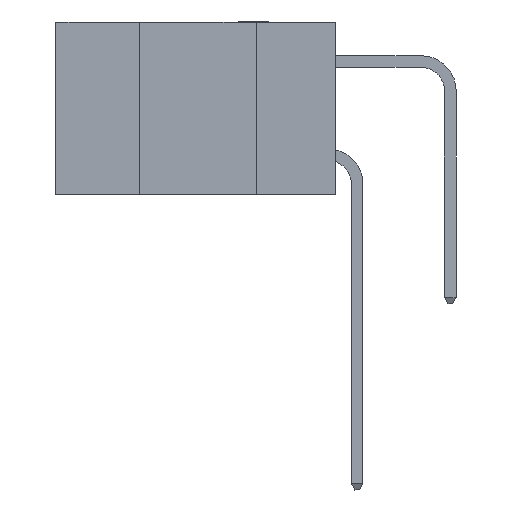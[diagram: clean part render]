
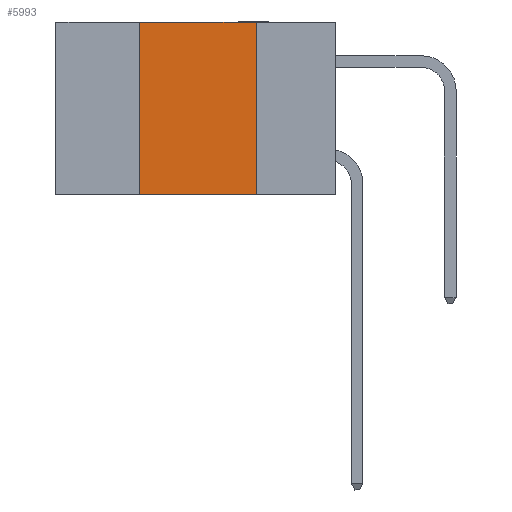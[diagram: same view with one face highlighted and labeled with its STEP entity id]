
A CAD part, left-side view. The second image highlights one B-rep face of the part: STEP entity #5993.
In plain terms, the highlighted planar face has unit normal (-1, 0, 0).
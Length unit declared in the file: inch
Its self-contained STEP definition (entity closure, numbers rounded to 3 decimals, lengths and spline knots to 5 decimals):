
#5 = VECTOR ( 'NONE', #8102, 39.37008 ) ;
#407 = LINE ( 'NONE', #8889, #17826 ) ;
#636 = CARTESIAN_POINT ( 'NONE',  ( 0., 0.6, 0. ) ) ;
#2403 = DIRECTION ( 'NONE',  ( 1., 0., 0. ) ) ;
#3461 = DIRECTION ( 'NONE',  ( 0., 0., 1. ) ) ;
#4046 = CARTESIAN_POINT ( 'NONE',  ( 0., 0.42, 0. ) ) ;
#4615 = VERTEX_POINT ( 'NONE', #21338 ) ;
#4782 = LINE ( 'NONE', #7060, #22530 ) ;
#5993 = ADVANCED_FACE ( 'NONE', ( #9013 ), #21867, .F. ) ;
#6171 = DIRECTION ( 'NONE',  ( 0., -1., 0. ) ) ;
#7060 = CARTESIAN_POINT ( 'NONE',  ( 0., 0.17, 0. ) ) ;
#7502 = VECTOR ( 'NONE', #6171, 39.37008 ) ;
#8099 = VERTEX_POINT ( 'NONE', #4046 ) ;
#8102 = DIRECTION ( 'NONE',  ( 0., -1., 0. ) ) ;
#8628 = EDGE_CURVE ( 'NONE', #8099, #14065, #18560, .T. ) ;
#8889 = CARTESIAN_POINT ( 'NONE',  ( 0., 0.42, 0. ) ) ;
#9013 = FACE_OUTER_BOUND ( 'NONE', #13429, .T. ) ;
#9877 = ORIENTED_EDGE ( 'NONE', *, *, #11554, .F. ) ;
#11554 = EDGE_CURVE ( 'NONE', #14065, #4615, #4782, .T. ) ;
#13429 = EDGE_LOOP ( 'NONE', ( #9877, #17192, #20737, #22029 ) ) ;
#14065 = VERTEX_POINT ( 'NONE', #21586 ) ;
#14379 = DIRECTION ( 'NONE',  ( 0., 0., -1. ) ) ;
#15825 = CARTESIAN_POINT ( 'NONE',  ( 0., 0.42, -0.37 ) ) ;
#17192 = ORIENTED_EDGE ( 'NONE', *, *, #8628, .F. ) ;
#17826 = VECTOR ( 'NONE', #3461, 39.37008 ) ;
#18019 = VERTEX_POINT ( 'NONE', #15825 ) ;
#18371 = EDGE_CURVE ( 'NONE', #18019, #8099, #407, .T. ) ;
#18560 = LINE ( 'NONE', #20340, #7502 ) ;
#18673 = CARTESIAN_POINT ( 'NONE',  ( 0., 0.6, -0.37 ) ) ;
#19372 = LINE ( 'NONE', #18673, #5 ) ;
#20125 = DIRECTION ( 'NONE',  ( 0., 0., -1. ) ) ;
#20340 = CARTESIAN_POINT ( 'NONE',  ( 0., 0.6, 0. ) ) ;
#20737 = ORIENTED_EDGE ( 'NONE', *, *, #18371, .F. ) ;
#21338 = CARTESIAN_POINT ( 'NONE',  ( 0., 0.17, -0.37 ) ) ;
#21489 = AXIS2_PLACEMENT_3D ( 'NONE', #636, #2403, #20125 ) ;
#21586 = CARTESIAN_POINT ( 'NONE',  ( 0., 0.17, 0. ) ) ;
#21867 = PLANE ( 'NONE',  #21489 ) ;
#22029 = ORIENTED_EDGE ( 'NONE', *, *, #22283, .T. ) ;
#22283 = EDGE_CURVE ( 'NONE', #18019, #4615, #19372, .T. ) ;
#22530 = VECTOR ( 'NONE', #14379, 39.37008 ) ;
